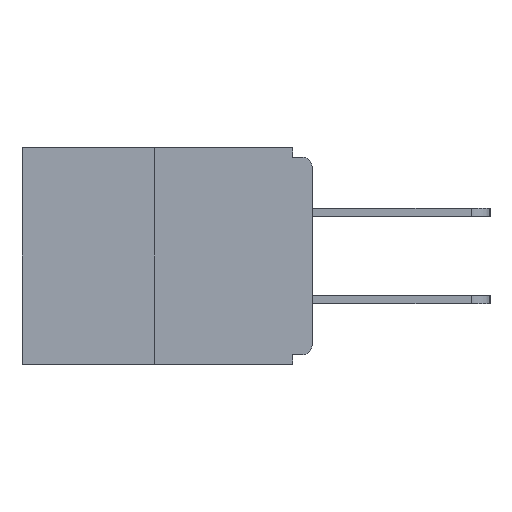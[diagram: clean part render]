
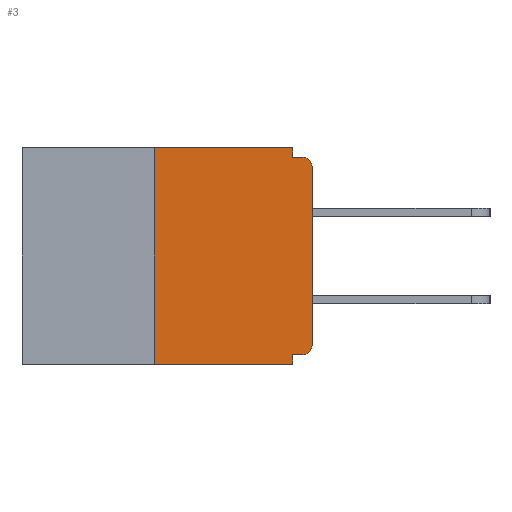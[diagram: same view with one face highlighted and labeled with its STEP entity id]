
A CAD part, left-side view. The second image highlights one B-rep face of the part: STEP entity #3.
In plain terms, the highlighted planar face has unit normal (-1, 0, 0).
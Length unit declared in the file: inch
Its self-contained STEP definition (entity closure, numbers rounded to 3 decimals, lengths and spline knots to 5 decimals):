
#3 = ADVANCED_FACE ( 'NONE', ( #7832 ), #6600, .F. ) ;
#178 = DIRECTION ( 'NONE',  ( 0., -1., 0. ) ) ;
#231 = DIRECTION ( 'NONE',  ( 1., 0., 0. ) ) ;
#241 = LINE ( 'NONE', #6399, #11084 ) ;
#526 = EDGE_CURVE ( 'NONE', #3743, #5875, #10616, .T. ) ;
#563 = ORIENTED_EDGE ( 'NONE', *, *, #19927, .F. ) ;
#967 = ORIENTED_EDGE ( 'NONE', *, *, #1977, .F. ) ;
#1222 = VERTEX_POINT ( 'NONE', #17162 ) ;
#1320 = CARTESIAN_POINT ( 'NONE',  ( 0., 0.25, 0. ) ) ;
#1550 = CARTESIAN_POINT ( 'NONE',  ( 0., 0.46, -0.343 ) ) ;
#1977 = EDGE_CURVE ( 'NONE', #5567, #1222, #9603, .T. ) ;
#2315 = EDGE_CURVE ( 'NONE', #19317, #18280, #2703, .T. ) ;
#2443 = VECTOR ( 'NONE', #178, 39.37008 ) ;
#2660 = LINE ( 'NONE', #1320, #8790 ) ;
#2703 = CIRCLE ( 'NONE', #4615, 0.015 ) ;
#2800 = VERTEX_POINT ( 'NONE', #5802 ) ;
#2810 = CARTESIAN_POINT ( 'NONE',  ( 0., 0.015, -0.03 ) ) ;
#3637 = ORIENTED_EDGE ( 'NONE', *, *, #15995, .F. ) ;
#3740 = CARTESIAN_POINT ( 'NONE',  ( 0., 0.015, -0.313 ) ) ;
#3743 = VERTEX_POINT ( 'NONE', #4911 ) ;
#4158 = DIRECTION ( 'NONE',  ( 0., 0., 1. ) ) ;
#4429 = CARTESIAN_POINT ( 'NONE',  ( 0., 0.031, 0. ) ) ;
#4615 = AXIS2_PLACEMENT_3D ( 'NONE', #2810, #16991, #12436 ) ;
#4911 = CARTESIAN_POINT ( 'NONE',  ( 0., 0.031, 0. ) ) ;
#5137 = CARTESIAN_POINT ( 'NONE',  ( 0., 0.015, -0.328 ) ) ;
#5147 = VECTOR ( 'NONE', #8999, 39.37008 ) ;
#5278 = VECTOR ( 'NONE', #13936, 39.37008 ) ;
#5567 = VERTEX_POINT ( 'NONE', #14406 ) ;
#5592 = VERTEX_POINT ( 'NONE', #5137 ) ;
#5725 = CARTESIAN_POINT ( 'NONE',  ( 0., 0., 0. ) ) ;
#5802 = CARTESIAN_POINT ( 'NONE',  ( 0., 0.25, -0.343 ) ) ;
#5859 = ORIENTED_EDGE ( 'NONE', *, *, #16945, .T. ) ;
#5875 = VERTEX_POINT ( 'NONE', #14085 ) ;
#6006 = CARTESIAN_POINT ( 'NONE',  ( 0., 0.25, 0. ) ) ;
#6399 = CARTESIAN_POINT ( 'NONE',  ( 0., 0., -0.328 ) ) ;
#6600 = PLANE ( 'NONE',  #7019 ) ;
#6916 = ORIENTED_EDGE ( 'NONE', *, *, #13078, .F. ) ;
#7019 = AXIS2_PLACEMENT_3D ( 'NONE', #14326, #231, #15745 ) ;
#7281 = LINE ( 'NONE', #16718, #5147 ) ;
#7373 = DIRECTION ( 'NONE',  ( 0., 0., -1. ) ) ;
#7536 = CIRCLE ( 'NONE', #13050, 0.015 ) ;
#7775 = LINE ( 'NONE', #13980, #2443 ) ;
#7832 = FACE_OUTER_BOUND ( 'NONE', #17523, .T. ) ;
#7897 = CARTESIAN_POINT ( 'NONE',  ( 0., 0.031, -0.343 ) ) ;
#8608 = DIRECTION ( 'NONE',  ( -1., 0., 0. ) ) ;
#8743 = CARTESIAN_POINT ( 'NONE',  ( 0., 0.015, -0.015 ) ) ;
#8790 = VECTOR ( 'NONE', #4158, 39.37008 ) ;
#8999 = DIRECTION ( 'NONE',  ( 0., -1., 0. ) ) ;
#9395 = VERTEX_POINT ( 'NONE', #18756 ) ;
#9603 = LINE ( 'NONE', #7897, #15311 ) ;
#9914 = DIRECTION ( 'NONE',  ( 0., 0., -1. ) ) ;
#10616 = LINE ( 'NONE', #4429, #17872 ) ;
#11084 = VECTOR ( 'NONE', #12605, 39.37008 ) ;
#11967 = VERTEX_POINT ( 'NONE', #6006 ) ;
#12248 = ORIENTED_EDGE ( 'NONE', *, *, #2315, .T. ) ;
#12365 = VECTOR ( 'NONE', #16392, 39.37008 ) ;
#12436 = DIRECTION ( 'NONE',  ( 0., 0., -1. ) ) ;
#12605 = DIRECTION ( 'NONE',  ( 0., 1., 0. ) ) ;
#12827 = ORIENTED_EDGE ( 'NONE', *, *, #526, .F. ) ;
#13050 = AXIS2_PLACEMENT_3D ( 'NONE', #3740, #8608, #9914 ) ;
#13078 = EDGE_CURVE ( 'NONE', #11967, #3743, #7281, .T. ) ;
#13936 = DIRECTION ( 'NONE',  ( 0., -1., 0. ) ) ;
#13980 = CARTESIAN_POINT ( 'NONE',  ( 0., 0., -0.015 ) ) ;
#14085 = CARTESIAN_POINT ( 'NONE',  ( 0., 0.031, -0.015 ) ) ;
#14321 = EDGE_CURVE ( 'NONE', #9395, #19317, #17897, .T. ) ;
#14326 = CARTESIAN_POINT ( 'NONE',  ( 0., 0.46, 0. ) ) ;
#14406 = CARTESIAN_POINT ( 'NONE',  ( 0., 0.031, -0.328 ) ) ;
#14725 = EDGE_CURVE ( 'NONE', #2800, #11967, #2660, .T. ) ;
#15311 = VECTOR ( 'NONE', #15608, 39.37008 ) ;
#15449 = LINE ( 'NONE', #1550, #5278 ) ;
#15608 = DIRECTION ( 'NONE',  ( 0., 0., -1. ) ) ;
#15745 = DIRECTION ( 'NONE',  ( 0., 0., -1. ) ) ;
#15900 = ORIENTED_EDGE ( 'NONE', *, *, #18026, .T. ) ;
#15995 = EDGE_CURVE ( 'NONE', #5592, #5567, #241, .T. ) ;
#16392 = DIRECTION ( 'NONE',  ( 0., 0., 1. ) ) ;
#16718 = CARTESIAN_POINT ( 'NONE',  ( 0., 0.46, 0. ) ) ;
#16945 = EDGE_CURVE ( 'NONE', #5592, #9395, #7536, .T. ) ;
#16991 = DIRECTION ( 'NONE',  ( -1., 0., 0. ) ) ;
#17162 = CARTESIAN_POINT ( 'NONE',  ( 0., 0.031, -0.343 ) ) ;
#17523 = EDGE_LOOP ( 'NONE', ( #6916, #18428, #15900, #967, #3637, #5859, #19612, #12248, #563, #12827 ) ) ;
#17872 = VECTOR ( 'NONE', #7373, 39.37008 ) ;
#17897 = LINE ( 'NONE', #5725, #12365 ) ;
#18026 = EDGE_CURVE ( 'NONE', #2800, #1222, #15449, .T. ) ;
#18271 = CARTESIAN_POINT ( 'NONE',  ( 0., 0., -0.03 ) ) ;
#18280 = VERTEX_POINT ( 'NONE', #8743 ) ;
#18428 = ORIENTED_EDGE ( 'NONE', *, *, #14725, .F. ) ;
#18756 = CARTESIAN_POINT ( 'NONE',  ( 0., 0., -0.313 ) ) ;
#19317 = VERTEX_POINT ( 'NONE', #18271 ) ;
#19612 = ORIENTED_EDGE ( 'NONE', *, *, #14321, .T. ) ;
#19927 = EDGE_CURVE ( 'NONE', #5875, #18280, #7775, .T. ) ;
